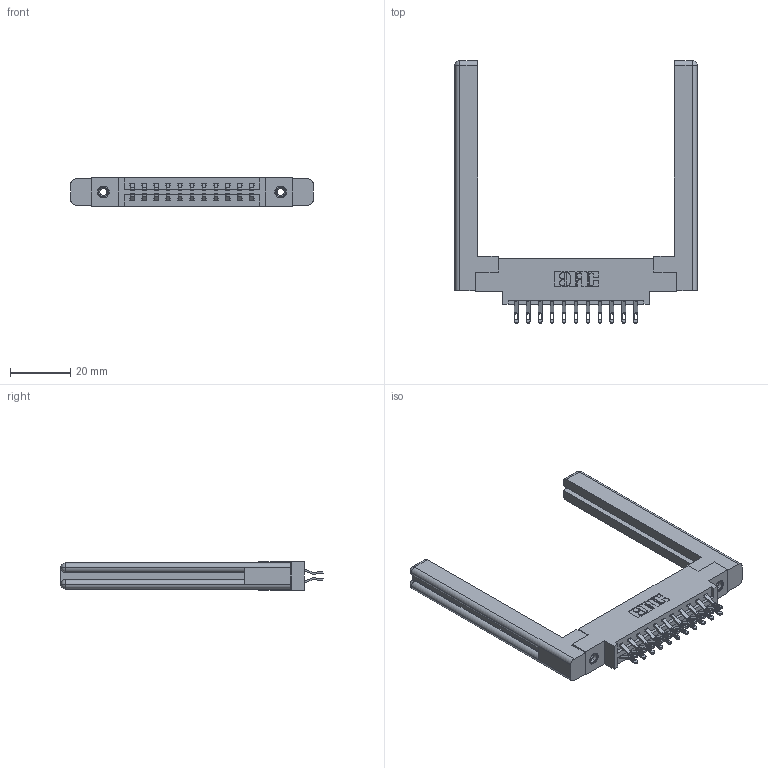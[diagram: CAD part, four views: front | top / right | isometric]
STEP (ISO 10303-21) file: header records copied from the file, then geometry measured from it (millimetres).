
FILE_DESCRIPTION (( 'STEP AP203' ), '1' );
FILE_NAME ('337-022-555-858.STEP', '2019-10-10T20:20:34', ( '' ), ( '' ), 'SwSTEP 2.0', 'SolidWorks 2016', '' );
FILE_SCHEMA (( 'CONFIG_CONTROL_DESIGN' ));
Length unit declared in the file: inch
Products named in the file (5): 307-220-058; 345-250-001_345-250-001-102; 337-022-555-858; 337 Part_0.170 Offset - 0.156 Dia-TI; 345-292-001_555 Tail
Assembly tree (27 placements, depth 2):
  337-022-555-858
    337 Part_0.170 Offset - 0.156 Dia-TI
    345-292-001_555 Tail  x22
    345-250-001_345-250-001-102  x2
    307-220-058  x2
Bounding box: 80.21 x 86.87 x 9.4 mm (x, y, z)
Volume: 15129.5 mm3; surface area: 14123.5 mm2
Topology: 27 solids, 27 shells, 1580 faces, 4835 edges, 3210 vertices
Faces by surface type: plane 950, cylinder 606, cone 12, torus 12
Entity records: 15630 total; most frequent: CARTESIAN_POINT 2703, ORIENTED_EDGE 2548, DIRECTION 2342, EDGE_CURVE 1274, VECTOR 1078, LINE 1078, VERTEX_POINT 842, AXIS2_PLACEMENT_3D 632
